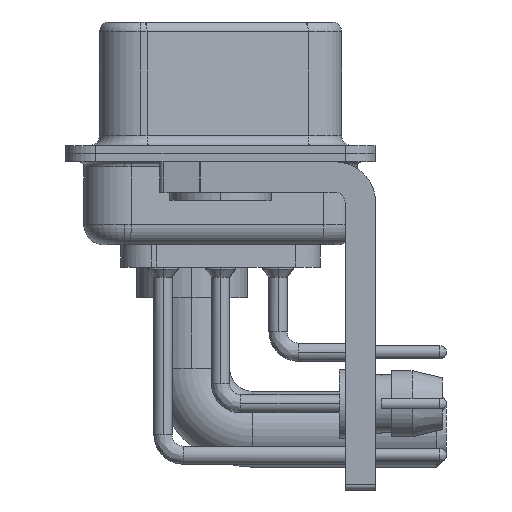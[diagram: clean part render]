
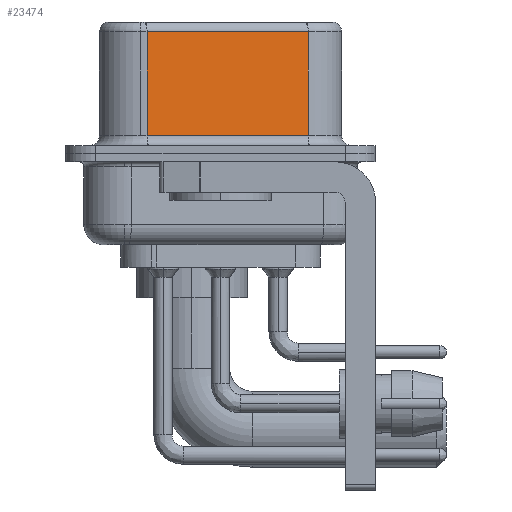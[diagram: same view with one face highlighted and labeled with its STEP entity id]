
A CAD part, left-side view. The second image highlights one B-rep face of the part: STEP entity #23474.
In plain terms, the highlighted planar face has unit normal (-0.985, -0.174, 0).
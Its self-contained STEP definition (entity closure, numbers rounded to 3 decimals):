
#1890 = ORIENTED_EDGE ( 'NONE', *, *, #22764, .T. ) ;
#1925 = VECTOR ( 'NONE', #37544, 1000. ) ;
#2636 = EDGE_CURVE ( 'NONE', #23566, #34853, #12999, .T. ) ;
#3941 = CARTESIAN_POINT ( 'NONE',  ( 5.132, -4.322, 6.52 ) ) ;
#4177 = VECTOR ( 'NONE', #32010, 1000. ) ;
#4902 = DIRECTION ( 'NONE',  ( -0.174, 0.985, 0. ) ) ;
#5558 = VERTEX_POINT ( 'NONE', #20499 ) ;
#5989 = ORIENTED_EDGE ( 'NONE', *, *, #2636, .F. ) ;
#6083 = CARTESIAN_POINT ( 'NONE',  ( 5.132, -4.322, 6.02 ) ) ;
#6138 = ORIENTED_EDGE ( 'NONE', *, *, #27165, .T. ) ;
#6221 = LINE ( 'NONE', #39643, #29556 ) ;
#8515 = DIRECTION ( 'NONE',  ( 0.985, 0.174, 0. ) ) ;
#11337 = FACE_OUTER_BOUND ( 'NONE', #19736, .T. ) ;
#12999 = LINE ( 'NONE', #3941, #1925 ) ;
#13208 = CARTESIAN_POINT ( 'NONE',  ( 3.73, 3.628, 6.02 ) ) ;
#14030 = VERTEX_POINT ( 'NONE', #13208 ) ;
#14034 = ORIENTED_EDGE ( 'NONE', *, *, #19174, .T. ) ;
#14208 = CARTESIAN_POINT ( 'NONE',  ( 5.132, -4.322, 0.9 ) ) ;
#16029 = DIRECTION ( 'NONE',  ( 0.174, -0.985, 0. ) ) ;
#16780 = PLANE ( 'NONE',  #32402 ) ;
#19174 = EDGE_CURVE ( 'NONE', #23566, #14030, #6221, .T. ) ;
#19736 = EDGE_LOOP ( 'NONE', ( #5989, #14034, #6138, #1890 ) ) ;
#20499 = CARTESIAN_POINT ( 'NONE',  ( 3.73, 3.628, 0.9 ) ) ;
#22764 = EDGE_CURVE ( 'NONE', #5558, #34853, #37564, .T. ) ;
#23474 = ADVANCED_FACE ( 'NONE', ( #11337 ), #16780, .F. ) ;
#23566 = VERTEX_POINT ( 'NONE', #6083 ) ;
#23608 = CARTESIAN_POINT ( 'NONE',  ( 5.132, -4.322, 6.52 ) ) ;
#24652 = VECTOR ( 'NONE', #16029, 1000. ) ;
#25686 = CARTESIAN_POINT ( 'NONE',  ( 5.132, -4.322, 0.9 ) ) ;
#27165 = EDGE_CURVE ( 'NONE', #14030, #5558, #28802, .T. ) ;
#28802 = LINE ( 'NONE', #32214, #4177 ) ;
#29556 = VECTOR ( 'NONE', #33793, 1000. ) ;
#32010 = DIRECTION ( 'NONE',  ( 0., 0., -1. ) ) ;
#32214 = CARTESIAN_POINT ( 'NONE',  ( 3.73, 3.628, 6.52 ) ) ;
#32402 = AXIS2_PLACEMENT_3D ( 'NONE', #23608, #8515, #4902 ) ;
#33793 = DIRECTION ( 'NONE',  ( -0.174, 0.985, 0. ) ) ;
#34853 = VERTEX_POINT ( 'NONE', #14208 ) ;
#37544 = DIRECTION ( 'NONE',  ( 0., 0., -1. ) ) ;
#37564 = LINE ( 'NONE', #25686, #24652 ) ;
#39643 = CARTESIAN_POINT ( 'NONE',  ( 5.132, -4.322, 6.02 ) ) ;
